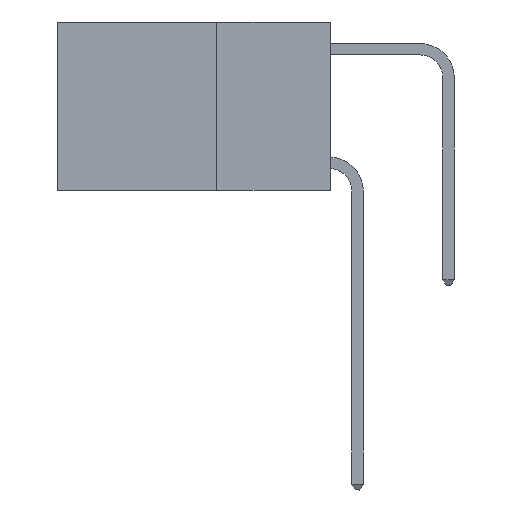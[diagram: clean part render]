
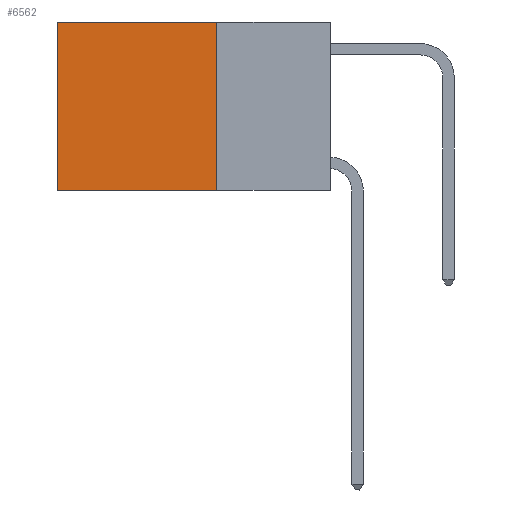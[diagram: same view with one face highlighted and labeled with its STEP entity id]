
A CAD part, left-side view. The second image highlights one B-rep face of the part: STEP entity #6562.
In plain terms, the highlighted planar face has unit normal (-1, 0, 0).
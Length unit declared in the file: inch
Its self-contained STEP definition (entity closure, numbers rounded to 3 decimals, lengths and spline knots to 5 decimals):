
#225 = CARTESIAN_POINT ( 'NONE',  ( 0.2625, 0.25, 0. ) ) ;
#4557 = VERTEX_POINT ( 'NONE', #27664 ) ;
#6562 = ADVANCED_FACE ( 'NONE', ( #15044 ), #13245, .F. ) ;
#7663 = CARTESIAN_POINT ( 'NONE',  ( 0.2625, 0.25, -0.37 ) ) ;
#8121 = DIRECTION ( 'NONE',  ( 0., 0., -1. ) ) ;
#8458 = CARTESIAN_POINT ( 'NONE',  ( 0.2625, 0.25, 0. ) ) ;
#8566 = VECTOR ( 'NONE', #29260, 39.37008 ) ;
#8693 = VECTOR ( 'NONE', #30969, 39.37008 ) ;
#9432 = VERTEX_POINT ( 'NONE', #14194 ) ;
#11138 = CARTESIAN_POINT ( 'NONE',  ( 0.2625, 0.25, 0. ) ) ;
#13129 = CARTESIAN_POINT ( 'NONE',  ( 0.2625, 0.6, 0. ) ) ;
#13182 = LINE ( 'NONE', #13129, #32943 ) ;
#13245 = PLANE ( 'NONE',  #20919 ) ;
#13556 = EDGE_LOOP ( 'NONE', ( #29382, #16871, #18104, #15932 ) ) ;
#14194 = CARTESIAN_POINT ( 'NONE',  ( 0.2625, 0.6, 0. ) ) ;
#15044 = FACE_OUTER_BOUND ( 'NONE', #13556, .T. ) ;
#15639 = CARTESIAN_POINT ( 'NONE',  ( 0.2625, 0.25, -0.37 ) ) ;
#15728 = DIRECTION ( 'NONE',  ( 0., 0., -1. ) ) ;
#15932 = ORIENTED_EDGE ( 'NONE', *, *, #19597, .T. ) ;
#16185 = DIRECTION ( 'NONE',  ( 0., 0., -1. ) ) ;
#16295 = LINE ( 'NONE', #11138, #8566 ) ;
#16871 = ORIENTED_EDGE ( 'NONE', *, *, #29564, .F. ) ;
#18104 = ORIENTED_EDGE ( 'NONE', *, *, #26218, .F. ) ;
#19497 = VERTEX_POINT ( 'NONE', #28923 ) ;
#19597 = EDGE_CURVE ( 'NONE', #19497, #9432, #16295, .T. ) ;
#20919 = AXIS2_PLACEMENT_3D ( 'NONE', #225, #23702, #8121 ) ;
#22559 = LINE ( 'NONE', #7663, #8693 ) ;
#23702 = DIRECTION ( 'NONE',  ( 1., 0., 0. ) ) ;
#24144 = VERTEX_POINT ( 'NONE', #15639 ) ;
#26218 = EDGE_CURVE ( 'NONE', #19497, #24144, #28753, .T. ) ;
#27664 = CARTESIAN_POINT ( 'NONE',  ( 0.2625, 0.6, -0.37 ) ) ;
#27948 = VECTOR ( 'NONE', #16185, 39.37008 ) ;
#28753 = LINE ( 'NONE', #8458, #27948 ) ;
#28923 = CARTESIAN_POINT ( 'NONE',  ( 0.2625, 0.25, 0. ) ) ;
#29260 = DIRECTION ( 'NONE',  ( 0., 1., 0. ) ) ;
#29382 = ORIENTED_EDGE ( 'NONE', *, *, #29616, .T. ) ;
#29564 = EDGE_CURVE ( 'NONE', #24144, #4557, #22559, .T. ) ;
#29616 = EDGE_CURVE ( 'NONE', #9432, #4557, #13182, .T. ) ;
#30969 = DIRECTION ( 'NONE',  ( 0., 1., 0. ) ) ;
#32943 = VECTOR ( 'NONE', #15728, 39.37008 ) ;
